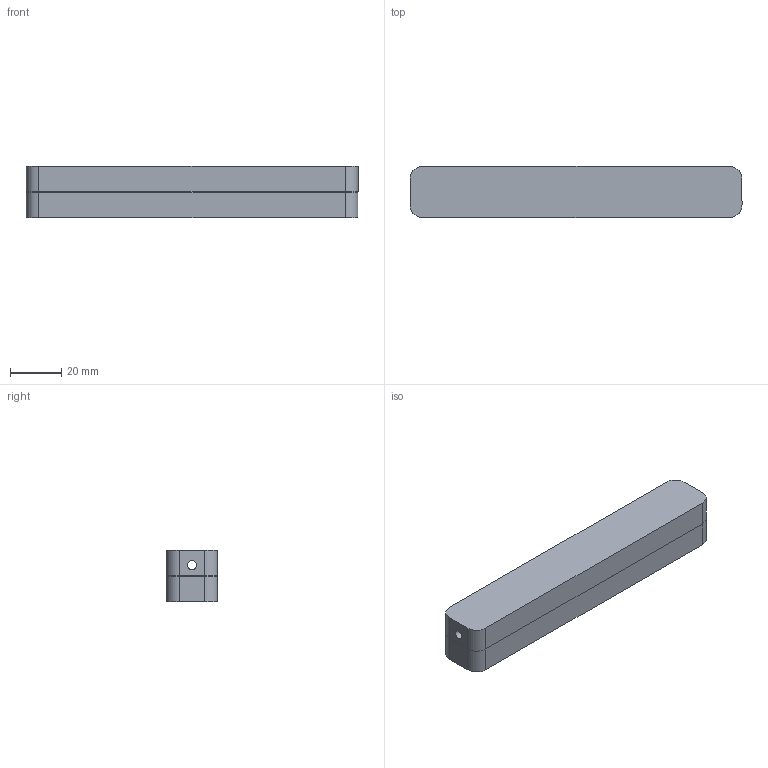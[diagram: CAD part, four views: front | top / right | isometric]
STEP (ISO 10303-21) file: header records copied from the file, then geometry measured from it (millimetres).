
FILE_DESCRIPTION(/* description */ (''),/* implementation_level */ '2;1');
FILE_NAME(/* name */ 'FGC-9_MkII_Drilling_Jig.step',/* time_stamp */ '2021-03-26T15:04:48+01:00',/* author */ (''),/* organization */ (''),/* preprocessor_version */ 'ST-DEVELOPER v18.1',/* originating_system */ 'Autodesk Translation Framework v9.10.0.1330',/* authorisation */ '');
FILE_SCHEMA (('AUTOMOTIVE_DESIGN { 1 0 10303 214 3 1 1 }'));
Length unit declared in the file: millimetre
Products named in the file (3): FGC-9_MkII_Drilling_Jig; Drilling Jig Hole Half; Drilling Jig Solid Half
Assembly tree (2 placements, depth 2):
  FGC-9_MkII_Drilling_Jig
    Drilling Jig Hole Half
    Drilling Jig Solid Half
Bounding box: 130 x 20 x 20 mm (x, y, z)
Volume: 37625 mm3; surface area: 18583.3 mm2
Topology: 2 solids, 2 shells, 28 faces, 66 edges, 44 vertices
Faces by surface type: plane 16, cylinder 12
Full cylindrical faces by diameter (mm): 3.6 x2
Entity records: 907 total; most frequent: DIRECTION 156, CARTESIAN_POINT 143, ORIENTED_EDGE 132, EDGE_CURVE 66, AXIS2_PLACEMENT_3D 57, VERTEX_POINT 44, LINE 42, VECTOR 42
